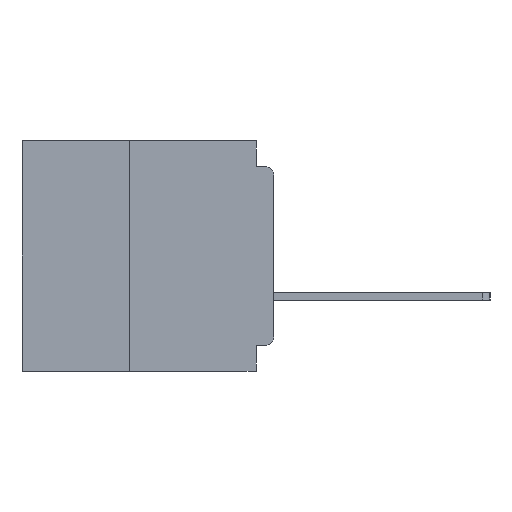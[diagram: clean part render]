
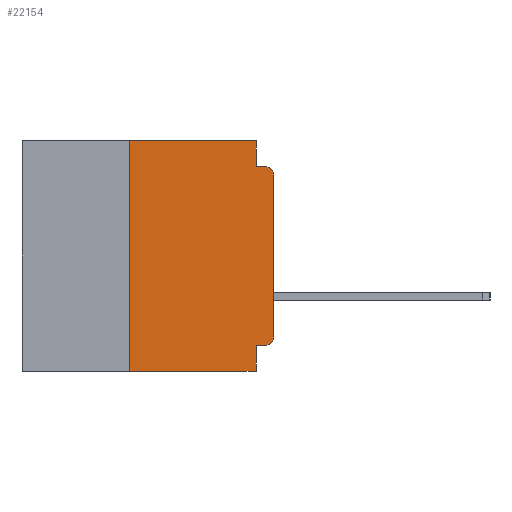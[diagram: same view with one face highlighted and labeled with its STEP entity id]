
A CAD part, left-side view. The second image highlights one B-rep face of the part: STEP entity #22154.
In plain terms, the highlighted planar face has unit normal (-1, 0, 0).
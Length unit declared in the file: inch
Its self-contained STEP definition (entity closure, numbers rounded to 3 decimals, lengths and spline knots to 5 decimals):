
#50 = CARTESIAN_POINT ( 'NONE',  ( 0., 0.031, -0.355 ) ) ;
#293 = ORIENTED_EDGE ( 'NONE', *, *, #13521, .F. ) ;
#375 = CARTESIAN_POINT ( 'NONE',  ( 0., 0., 0. ) ) ;
#672 = EDGE_CURVE ( 'NONE', #33433, #29879, #46705, .T. ) ;
#822 = DIRECTION ( 'NONE',  ( 0., 0., -1. ) ) ;
#3523 = EDGE_CURVE ( 'NONE', #13219, #52740, #37007, .T. ) ;
#4576 = LINE ( 'NONE', #42455, #38902 ) ;
#4936 = EDGE_CURVE ( 'NONE', #24300, #51912, #4576, .T. ) ;
#5856 = AXIS2_PLACEMENT_3D ( 'NONE', #9612, #40855, #14068 ) ;
#6611 = ORIENTED_EDGE ( 'NONE', *, *, #27177, .T. ) ;
#7190 = CARTESIAN_POINT ( 'NONE',  ( 0., 0.015, -0.355 ) ) ;
#7528 = VECTOR ( 'NONE', #45907, 39.37008 ) ;
#9208 = DIRECTION ( 'NONE',  ( 0., 0., 1. ) ) ;
#9612 = CARTESIAN_POINT ( 'NONE',  ( 0., 0.015, -0.34 ) ) ;
#10253 = EDGE_CURVE ( 'NONE', #52740, #13307, #14221, .T. ) ;
#12910 = CARTESIAN_POINT ( 'NONE',  ( 0., 0.015, -0.06 ) ) ;
#13219 = VERTEX_POINT ( 'NONE', #29740 ) ;
#13307 = VERTEX_POINT ( 'NONE', #30711 ) ;
#13521 = EDGE_CURVE ( 'NONE', #35781, #46731, #29939, .T. ) ;
#14068 = DIRECTION ( 'NONE',  ( 0., 0., -1. ) ) ;
#14221 = CIRCLE ( 'NONE', #54373, 0.015 ) ;
#17432 = DIRECTION ( 'NONE',  ( 0., 0., -1. ) ) ;
#19605 = VECTOR ( 'NONE', #33471, 39.37008 ) ;
#20646 = EDGE_CURVE ( 'NONE', #46731, #24300, #29306, .T. ) ;
#22154 = ADVANCED_FACE ( 'NONE', ( #55489 ), #27439, .F. ) ;
#22914 = VECTOR ( 'NONE', #51850, 39.37008 ) ;
#23711 = VECTOR ( 'NONE', #9208, 39.37008 ) ;
#24252 = CARTESIAN_POINT ( 'NONE',  ( 0., 0., -0.06 ) ) ;
#24300 = VERTEX_POINT ( 'NONE', #25835 ) ;
#24383 = LINE ( 'NONE', #46872, #32082 ) ;
#24628 = CARTESIAN_POINT ( 'NONE',  ( 0., 0.437, 0. ) ) ;
#24950 = AXIS2_PLACEMENT_3D ( 'NONE', #31959, #27619, #822 ) ;
#25835 = CARTESIAN_POINT ( 'NONE',  ( 0., 0.031, 0. ) ) ;
#26896 = CARTESIAN_POINT ( 'NONE',  ( 0., 0.031, -0.045 ) ) ;
#27177 = EDGE_CURVE ( 'NONE', #35781, #29879, #24383, .T. ) ;
#27241 = CARTESIAN_POINT ( 'NONE',  ( 0., 0.25, 0. ) ) ;
#27439 = PLANE ( 'NONE',  #24950 ) ;
#27619 = DIRECTION ( 'NONE',  ( 1., 0., 0. ) ) ;
#27870 = VECTOR ( 'NONE', #51408, 39.37008 ) ;
#28932 = CIRCLE ( 'NONE', #5856, 0.015 ) ;
#29102 = CARTESIAN_POINT ( 'NONE',  ( 0., 0., -0.045 ) ) ;
#29306 = LINE ( 'NONE', #24628, #27870 ) ;
#29573 = CARTESIAN_POINT ( 'NONE',  ( 0., 0.031, -0.4 ) ) ;
#29740 = CARTESIAN_POINT ( 'NONE',  ( 0., 0., -0.34 ) ) ;
#29879 = VERTEX_POINT ( 'NONE', #44120 ) ;
#29939 = LINE ( 'NONE', #41374, #7528 ) ;
#30711 = CARTESIAN_POINT ( 'NONE',  ( 0., 0.015, -0.045 ) ) ;
#31506 = LINE ( 'NONE', #33267, #19605 ) ;
#31959 = CARTESIAN_POINT ( 'NONE',  ( 0., 0.437, 0. ) ) ;
#32082 = VECTOR ( 'NONE', #51375, 39.37008 ) ;
#32391 = ORIENTED_EDGE ( 'NONE', *, *, #10253, .T. ) ;
#32536 = ORIENTED_EDGE ( 'NONE', *, *, #672, .F. ) ;
#33267 = CARTESIAN_POINT ( 'NONE',  ( 0., 0., -0.355 ) ) ;
#33433 = VERTEX_POINT ( 'NONE', #50 ) ;
#33471 = DIRECTION ( 'NONE',  ( 0., 1., 0. ) ) ;
#35781 = VERTEX_POINT ( 'NONE', #57855 ) ;
#36142 = EDGE_CURVE ( 'NONE', #55768, #33433, #31506, .T. ) ;
#36326 = ORIENTED_EDGE ( 'NONE', *, *, #36142, .F. ) ;
#37007 = LINE ( 'NONE', #375, #23711 ) ;
#38019 = ORIENTED_EDGE ( 'NONE', *, *, #45872, .F. ) ;
#38774 = VECTOR ( 'NONE', #56255, 39.37008 ) ;
#38902 = VECTOR ( 'NONE', #46983, 39.37008 ) ;
#40855 = DIRECTION ( 'NONE',  ( -1., 0., 0. ) ) ;
#41374 = CARTESIAN_POINT ( 'NONE',  ( 0., 0.25, -0.4 ) ) ;
#41531 = ORIENTED_EDGE ( 'NONE', *, *, #52586, .T. ) ;
#42383 = EDGE_LOOP ( 'NONE', ( #43004, #32391, #38019, #52980, #55156, #293, #6611, #32536, #36326, #41531 ) ) ;
#42455 = CARTESIAN_POINT ( 'NONE',  ( 0., 0.031, 0. ) ) ;
#43004 = ORIENTED_EDGE ( 'NONE', *, *, #3523, .T. ) ;
#44120 = CARTESIAN_POINT ( 'NONE',  ( 0., 0.031, -0.4 ) ) ;
#44196 = DIRECTION ( 'NONE',  ( -1., 0., 0. ) ) ;
#45872 = EDGE_CURVE ( 'NONE', #51912, #13307, #50675, .T. ) ;
#45907 = DIRECTION ( 'NONE',  ( 0., 0., 1. ) ) ;
#46705 = LINE ( 'NONE', #29573, #22914 ) ;
#46731 = VERTEX_POINT ( 'NONE', #27241 ) ;
#46872 = CARTESIAN_POINT ( 'NONE',  ( 0., 0.437, -0.4 ) ) ;
#46983 = DIRECTION ( 'NONE',  ( 0., 0., -1. ) ) ;
#50675 = LINE ( 'NONE', #29102, #38774 ) ;
#51375 = DIRECTION ( 'NONE',  ( 0., -1., 0. ) ) ;
#51408 = DIRECTION ( 'NONE',  ( 0., -1., 0. ) ) ;
#51850 = DIRECTION ( 'NONE',  ( 0., 0., -1. ) ) ;
#51912 = VERTEX_POINT ( 'NONE', #26896 ) ;
#52586 = EDGE_CURVE ( 'NONE', #55768, #13219, #28932, .T. ) ;
#52740 = VERTEX_POINT ( 'NONE', #24252 ) ;
#52980 = ORIENTED_EDGE ( 'NONE', *, *, #4936, .F. ) ;
#54373 = AXIS2_PLACEMENT_3D ( 'NONE', #12910, #44196, #17432 ) ;
#55156 = ORIENTED_EDGE ( 'NONE', *, *, #20646, .F. ) ;
#55489 = FACE_OUTER_BOUND ( 'NONE', #42383, .T. ) ;
#55768 = VERTEX_POINT ( 'NONE', #7190 ) ;
#56255 = DIRECTION ( 'NONE',  ( 0., -1., 0. ) ) ;
#57855 = CARTESIAN_POINT ( 'NONE',  ( 0., 0.25, -0.4 ) ) ;
